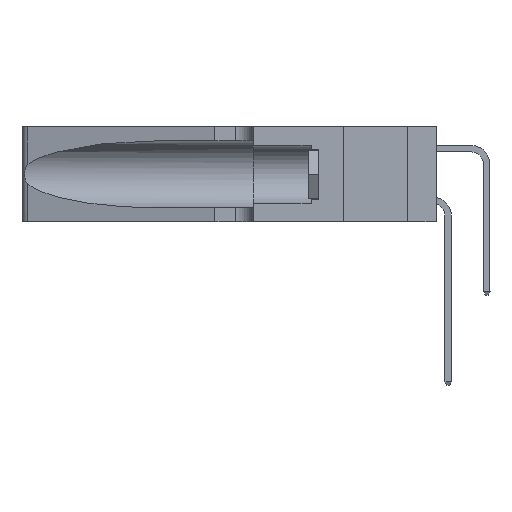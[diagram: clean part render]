
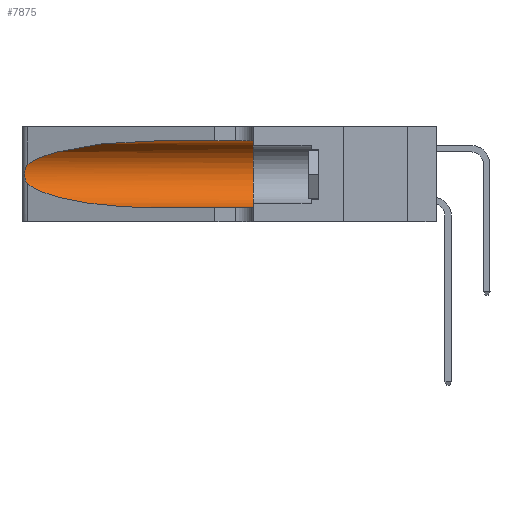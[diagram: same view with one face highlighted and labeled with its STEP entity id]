
A CAD part, left-side view. The second image highlights one B-rep face of the part: STEP entity #7875.
In plain terms, the highlighted cylindrical face has radius 3.308 mm (diameter 6.617 mm), a partial arc.
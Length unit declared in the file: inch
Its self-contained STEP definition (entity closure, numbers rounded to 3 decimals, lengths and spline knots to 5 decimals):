
#620 = CARTESIAN_POINT ( 'NONE',  ( 0.25639, 1.23186, 0.15144 ) ) ;
#726 = VERTEX_POINT ( 'NONE', #12784 ) ;
#768 = CARTESIAN_POINT ( 'NONE',  ( 0.1305, 0.72297, 0.05475 ) ) ;
#1890 = VERTEX_POINT ( 'NONE', #17591 ) ;
#1971 = EDGE_CURVE ( 'NONE', #5471, #16210, #9750, .T. ) ;
#2263 = EDGE_CURVE ( 'NONE', #16210, #726, #15421, .T. ) ;
#3119 = ORIENTED_EDGE ( 'NONE', *, *, #2263, .T. ) ;
#3633 = CARTESIAN_POINT ( 'NONE',  ( 0.25856, 1.23593, 0.16098 ) ) ;
#3656 = ORIENTED_EDGE ( 'NONE', *, *, #1971, .T. ) ;
#4249 = CARTESIAN_POINT ( 'NONE',  ( 0.1305, 1.61858, 0.05475 ) ) ;
#4293 = EDGE_CURVE ( 'NONE', #726, #17182, #20035, .T. ) ;
#4554 =( BOUNDED_CURVE ( )  B_SPLINE_CURVE ( 3, ( #11609, #18320, #16438, #18117 ),
 .UNSPECIFIED., .F., .T. ) 
 B_SPLINE_CURVE_WITH_KNOTS ( ( 4, 4 ),
 ( 1.5708, 2.84003 ),
 .UNSPECIFIED. ) 
 CURVE ( )  GEOMETRIC_REPRESENTATION_ITEM ( )  RATIONAL_B_SPLINE_CURVE ( ( 1., 0.87, 0.87, 1. ) ) 
 REPRESENTATION_ITEM ( '' )  );
#4885 = EDGE_LOOP ( 'NONE', ( #18871, #3656, #3119, #19406, #15002, #6541 ) ) ;
#5471 = VERTEX_POINT ( 'NONE', #8228 ) ;
#5510 = CARTESIAN_POINT ( 'NONE',  ( 0.25487, 1.22718, 0.14631 ) ) ;
#6197 = CARTESIAN_POINT ( 'NONE',  ( 0.25487, 1.22718, 0.14631 ) ) ;
#6205 = EDGE_CURVE ( 'NONE', #1890, #12873, #17504, .T. ) ;
#6322 = EDGE_CURVE ( 'NONE', #12873, #17182, #8715, .T. ) ;
#6436 = CYLINDRICAL_SURFACE ( 'NONE', #20543, 0.13025 ) ;
#6541 = ORIENTED_EDGE ( 'NONE', *, *, #6205, .F. ) ;
#7553 = VECTOR ( 'NONE', #18601, 39.37008 ) ;
#7875 = ADVANCED_FACE ( 'NONE', ( #11163 ), #6436, .F. ) ;
#8228 = CARTESIAN_POINT ( 'NONE',  ( 0.25487, 1.22718, 0.22369 ) ) ;
#8272 = CARTESIAN_POINT ( 'NONE',  ( 0.26075, 1.23896, 0.19203 ) ) ;
#8407 = CARTESIAN_POINT ( 'NONE',  ( 0.25789, 1.23486, 0.15765 ) ) ;
#8469 = VECTOR ( 'NONE', #13149, 39.37008 ) ;
#8534 = DIRECTION ( 'NONE',  ( 0., 0., -1. ) ) ;
#8543 = DIRECTION ( 'NONE',  ( 0., 1., 0. ) ) ;
#8715 = CIRCLE ( 'NONE', #15445, 0.13025 ) ;
#9750 = B_SPLINE_CURVE_WITH_KNOTS ( 'NONE', 3,
 ( #14916, #11683, #16389, #11548, #13137, #17855, #8272, #19733, #10145, #3633, #8407, #620, #19597, #9862 ),
 .UNSPECIFIED., .F., .F.,
 ( 4, 2, 2, 2, 2, 2, 4 ),
 ( 0., 0.00027, 0.00053, 0.00107, 0.0016, 0.00187, 0.00214 ),
 .UNSPECIFIED. ) ;
#9862 = CARTESIAN_POINT ( 'NONE',  ( 0.25487, 1.22718, 0.14631 ) ) ;
#10145 = CARTESIAN_POINT ( 'NONE',  ( 0.26017, 1.23833, 0.17102 ) ) ;
#10276 = CARTESIAN_POINT ( 'NONE',  ( 0.1305, 0.35, 0.185 ) ) ;
#10298 = CARTESIAN_POINT ( 'NONE',  ( 0.2373, 1.15595, 0.08982 ) ) ;
#11163 = FACE_OUTER_BOUND ( 'NONE', #4885, .T. ) ;
#11548 = CARTESIAN_POINT ( 'NONE',  ( 0.25787, 1.23484, 0.2124 ) ) ;
#11559 = CARTESIAN_POINT ( 'NONE',  ( 0.1305, 1.61858, 0.31525 ) ) ;
#11609 = CARTESIAN_POINT ( 'NONE',  ( 0.1305, 0.72297, 0.31525 ) ) ;
#11683 = CARTESIAN_POINT ( 'NONE',  ( 0.25555, 1.22994, 0.2215 ) ) ;
#12784 = CARTESIAN_POINT ( 'NONE',  ( 0.1305, 0.72297, 0.05475 ) ) ;
#12873 = VERTEX_POINT ( 'NONE', #20287 ) ;
#13137 = CARTESIAN_POINT ( 'NONE',  ( 0.25854, 1.2359, 0.20912 ) ) ;
#13149 = DIRECTION ( 'NONE',  ( 0., -1., 0. ) ) ;
#14916 = CARTESIAN_POINT ( 'NONE',  ( 0.25487, 1.22718, 0.22369 ) ) ;
#15002 = ORIENTED_EDGE ( 'NONE', *, *, #6322, .F. ) ;
#15038 = DIRECTION ( 'NONE',  ( 0., -1., 0. ) ) ;
#15373 = EDGE_CURVE ( 'NONE', #1890, #5471, #4554, .T. ) ;
#15421 =( BOUNDED_CURVE ( )  B_SPLINE_CURVE ( 3, ( #5510, #10298, #16745, #768 ),
 .UNSPECIFIED., .F., .F. ) 
 B_SPLINE_CURVE_WITH_KNOTS ( ( 4, 4 ),
 ( 3.44316, 4.71239 ),
 .UNSPECIFIED. ) 
 CURVE ( )  GEOMETRIC_REPRESENTATION_ITEM ( )  RATIONAL_B_SPLINE_CURVE ( ( 1., 0.87, 0.87, 1. ) ) 
 REPRESENTATION_ITEM ( '' )  );
#15445 = AXIS2_PLACEMENT_3D ( 'NONE', #10276, #8543, #16515 ) ;
#16210 = VERTEX_POINT ( 'NONE', #6197 ) ;
#16389 = CARTESIAN_POINT ( 'NONE',  ( 0.25639, 1.23184, 0.21858 ) ) ;
#16438 = CARTESIAN_POINT ( 'NONE',  ( 0.2373, 1.15595, 0.28018 ) ) ;
#16515 = DIRECTION ( 'NONE',  ( 0., 0., 1. ) ) ;
#16745 = CARTESIAN_POINT ( 'NONE',  ( 0.18966, 0.96281, 0.05475 ) ) ;
#17182 = VERTEX_POINT ( 'NONE', #18514 ) ;
#17504 = LINE ( 'NONE', #11559, #8469 ) ;
#17591 = CARTESIAN_POINT ( 'NONE',  ( 0.1305, 0.72297, 0.31525 ) ) ;
#17855 = CARTESIAN_POINT ( 'NONE',  ( 0.26018, 1.23835, 0.19895 ) ) ;
#17971 = CARTESIAN_POINT ( 'NONE',  ( 0.1305, 1.61858, 0.185 ) ) ;
#18117 = CARTESIAN_POINT ( 'NONE',  ( 0.25487, 1.22718, 0.22369 ) ) ;
#18320 = CARTESIAN_POINT ( 'NONE',  ( 0.18966, 0.96281, 0.31525 ) ) ;
#18514 = CARTESIAN_POINT ( 'NONE',  ( 0.1305, 0.35, 0.05475 ) ) ;
#18601 = DIRECTION ( 'NONE',  ( 0., -1., 0. ) ) ;
#18871 = ORIENTED_EDGE ( 'NONE', *, *, #15373, .T. ) ;
#19406 = ORIENTED_EDGE ( 'NONE', *, *, #4293, .T. ) ;
#19597 = CARTESIAN_POINT ( 'NONE',  ( 0.25555, 1.22993, 0.14849 ) ) ;
#19733 = CARTESIAN_POINT ( 'NONE',  ( 0.26075, 1.23896, 0.178 ) ) ;
#20035 = LINE ( 'NONE', #4249, #7553 ) ;
#20287 = CARTESIAN_POINT ( 'NONE',  ( 0.1305, 0.35, 0.31525 ) ) ;
#20543 = AXIS2_PLACEMENT_3D ( 'NONE', #17971, #15038, #8534 ) ;
